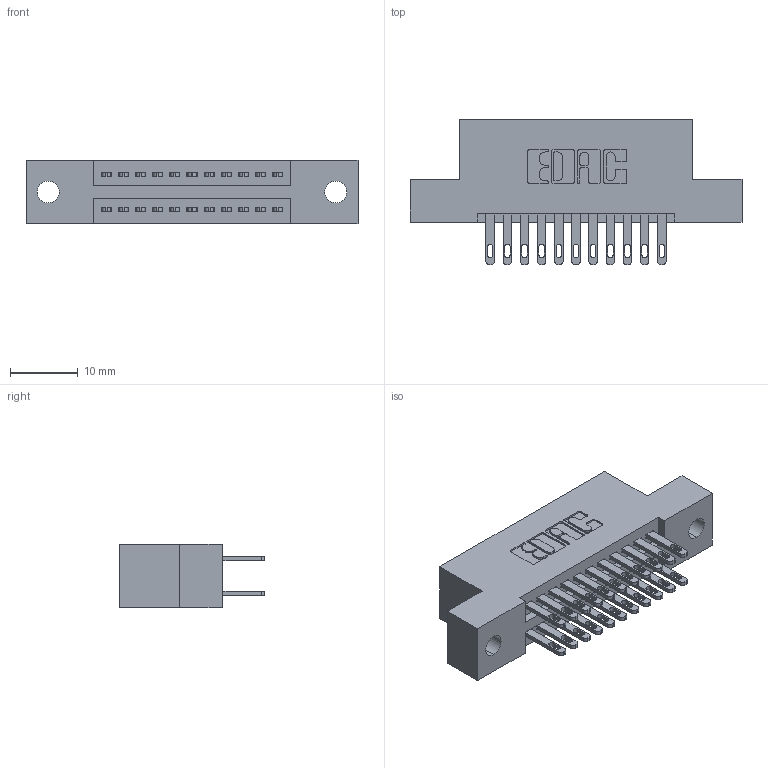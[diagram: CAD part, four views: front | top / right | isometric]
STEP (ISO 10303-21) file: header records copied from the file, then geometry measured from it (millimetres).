
FILE_DESCRIPTION (( 'STEP AP203' ), '1' );
FILE_NAME ('345-022-500-202.STEP', '2018-08-20T10:34:47', ( '' ), ( '' ), 'SwSTEP 2.0', 'SolidWorks 2016', '' );
FILE_SCHEMA (( 'CONFIG_CONTROL_DESIGN' ));
Length unit declared in the file: inch
Products named in the file (3): 345 Part_Flush Mounting Lugs - 0.128 Dia; 345-292-001_345-293-100; 345-022-500-202
Assembly tree (23 placements, depth 2):
  345-022-500-202
    345 Part_Flush Mounting Lugs - 0.128 Dia
    345-292-001_345-293-100  x22
Bounding box: 49.15 x 21.51 x 9.4 mm (x, y, z)
Volume: 4517.2 mm3; surface area: 6028.4 mm2
Topology: 23 solids, 23 shells, 1138 faces, 3443 edges, 2294 vertices
Faces by surface type: plane 674, cylinder 464
Entity records: 12737 total; most frequent: CARTESIAN_POINT 2164, ORIENTED_EDGE 2098, DIRECTION 1949, EDGE_CURVE 1049, VECTOR 869, LINE 869, VERTEX_POINT 698, AXIS2_PLACEMENT_3D 540
